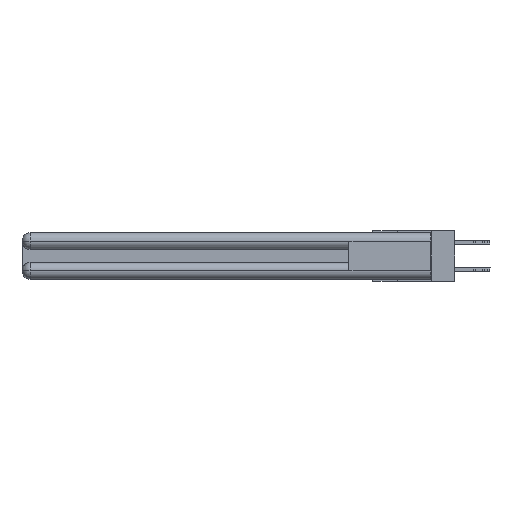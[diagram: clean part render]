
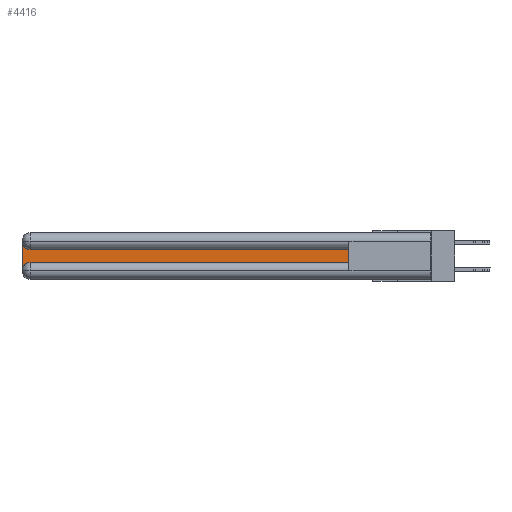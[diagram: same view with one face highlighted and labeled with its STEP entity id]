
A CAD part, left-side view. The second image highlights one B-rep face of the part: STEP entity #4416.
In plain terms, the highlighted planar face has unit normal (-1, 0, 0).
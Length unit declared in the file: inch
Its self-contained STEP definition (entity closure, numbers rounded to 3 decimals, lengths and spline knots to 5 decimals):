
#98 = CARTESIAN_POINT ( 'NONE',  ( 0.075, 0.6, -0.1225 ) ) ;
#133 = DIRECTION ( 'NONE',  ( 1., 0., 0. ) ) ;
#1246 = AXIS2_PLACEMENT_3D ( 'NONE', #9547, #16546, #11803 ) ;
#1357 = VERTEX_POINT ( 'NONE', #22836 ) ;
#1738 = VECTOR ( 'NONE', #22442, 39.37008 ) ;
#1970 = EDGE_CURVE ( 'NONE', #7348, #1357, #12618, .T. ) ;
#2239 = CARTESIAN_POINT ( 'NONE',  ( 0.075, 2.94, -0.1225 ) ) ;
#2428 = CARTESIAN_POINT ( 'NONE',  ( 0.075, 3., -0.2775 ) ) ;
#4160 = EDGE_CURVE ( 'NONE', #1357, #14573, #14680, .T. ) ;
#4399 = DIRECTION ( 'NONE',  ( 0., 0., -1. ) ) ;
#4416 = ADVANCED_FACE ( 'NONE', ( #12066 ), #18738, .F. ) ;
#4960 = VECTOR ( 'NONE', #7440, 39.37008 ) ;
#5086 = EDGE_CURVE ( 'NONE', #16583, #7348, #15355, .T. ) ;
#5453 = EDGE_CURVE ( 'NONE', #14573, #16537, #5722, .T. ) ;
#5526 = ORIENTED_EDGE ( 'NONE', *, *, #5453, .T. ) ;
#5647 = EDGE_CURVE ( 'NONE', #16537, #12108, #19448, .T. ) ;
#5648 = CARTESIAN_POINT ( 'NONE',  ( 0.075, 0.6, -0.2175 ) ) ;
#5722 = LINE ( 'NONE', #98, #4960 ) ;
#6501 = VECTOR ( 'NONE', #26201, 39.37008 ) ;
#6591 = CARTESIAN_POINT ( 'NONE',  ( 0.075, 3., -0.2175 ) ) ;
#7348 = VERTEX_POINT ( 'NONE', #10889 ) ;
#7422 = ORIENTED_EDGE ( 'NONE', *, *, #5086, .T. ) ;
#7440 = DIRECTION ( 'NONE',  ( 0., 1., 0. ) ) ;
#7534 = EDGE_CURVE ( 'NONE', #12108, #16583, #19124, .T. ) ;
#7979 = ORIENTED_EDGE ( 'NONE', *, *, #1970, .T. ) ;
#7981 = CARTESIAN_POINT ( 'NONE',  ( 0.075, 0.6, -0.1225 ) ) ;
#9547 = CARTESIAN_POINT ( 'NONE',  ( 0.075, 3., -0.1225 ) ) ;
#10889 = CARTESIAN_POINT ( 'NONE',  ( 0.075, 2.94, -0.2175 ) ) ;
#11362 = EDGE_LOOP ( 'NONE', ( #5526, #23786, #25333, #7422, #7979, #27434 ) ) ;
#11487 = CARTESIAN_POINT ( 'NONE',  ( 0.075, 3., -0.0625 ) ) ;
#11803 = DIRECTION ( 'NONE',  ( 0., 0., -1. ) ) ;
#11849 = VECTOR ( 'NONE', #27050, 39.37008 ) ;
#12066 = FACE_OUTER_BOUND ( 'NONE', #11362, .T. ) ;
#12108 = VERTEX_POINT ( 'NONE', #11487 ) ;
#12618 = LINE ( 'NONE', #15142, #11849 ) ;
#14573 = VERTEX_POINT ( 'NONE', #7981 ) ;
#14680 = LINE ( 'NONE', #5648, #1738 ) ;
#15142 = CARTESIAN_POINT ( 'NONE',  ( 0.075, 0.6, -0.2175 ) ) ;
#15355 = CIRCLE ( 'NONE', #22325, 0.06 ) ;
#16153 = CARTESIAN_POINT ( 'NONE',  ( 0.075, 2.94, -0.0625 ) ) ;
#16537 = VERTEX_POINT ( 'NONE', #2239 ) ;
#16546 = DIRECTION ( 'NONE',  ( 1., 0., 0. ) ) ;
#16583 = VERTEX_POINT ( 'NONE', #2428 ) ;
#16755 = DIRECTION ( 'NONE',  ( 0., 0., -1. ) ) ;
#18558 = DIRECTION ( 'NONE',  ( 1., 0., 0. ) ) ;
#18738 = PLANE ( 'NONE',  #1246 ) ;
#18930 = CARTESIAN_POINT ( 'NONE',  ( 0.075, 2.94, -0.2775 ) ) ;
#19124 = LINE ( 'NONE', #6591, #6501 ) ;
#19448 = CIRCLE ( 'NONE', #28718, 0.06 ) ;
#22325 = AXIS2_PLACEMENT_3D ( 'NONE', #18930, #133, #16755 ) ;
#22442 = DIRECTION ( 'NONE',  ( 0., 0., 1. ) ) ;
#22836 = CARTESIAN_POINT ( 'NONE',  ( 0.075, 0.6, -0.2175 ) ) ;
#23786 = ORIENTED_EDGE ( 'NONE', *, *, #5647, .T. ) ;
#25333 = ORIENTED_EDGE ( 'NONE', *, *, #7534, .T. ) ;
#26201 = DIRECTION ( 'NONE',  ( 0., 0., -1. ) ) ;
#27050 = DIRECTION ( 'NONE',  ( 0., -1., 0. ) ) ;
#27434 = ORIENTED_EDGE ( 'NONE', *, *, #4160, .T. ) ;
#28718 = AXIS2_PLACEMENT_3D ( 'NONE', #16153, #18558, #4399 ) ;
